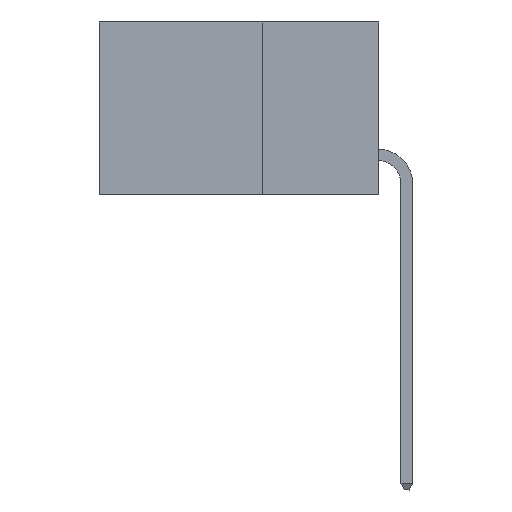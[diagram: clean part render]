
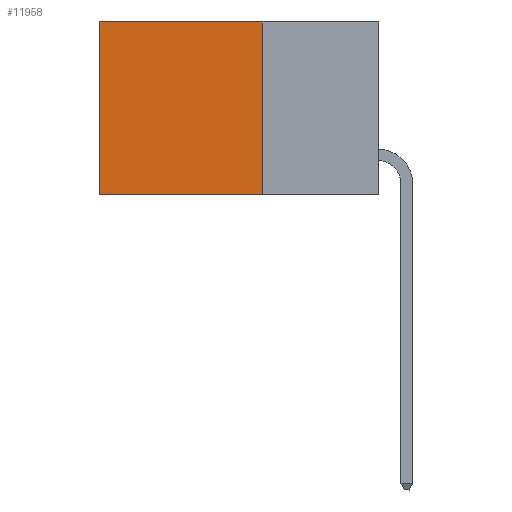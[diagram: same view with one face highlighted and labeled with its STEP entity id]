
A CAD part, left-side view. The second image highlights one B-rep face of the part: STEP entity #11958.
In plain terms, the highlighted planar face has unit normal (-1, 0, 0).
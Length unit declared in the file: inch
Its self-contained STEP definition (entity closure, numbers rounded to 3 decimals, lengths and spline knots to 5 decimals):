
#182 = DIRECTION ( 'NONE',  ( 0., 0., -1. ) ) ;
#1969 = CARTESIAN_POINT ( 'NONE',  ( 0.298, 0.25, -0.37 ) ) ;
#2810 = LINE ( 'NONE', #8745, #17818 ) ;
#3783 = CARTESIAN_POINT ( 'NONE',  ( 0.298, 0.25, 0. ) ) ;
#4049 = DIRECTION ( 'NONE',  ( 0., 1., 0. ) ) ;
#4136 = CARTESIAN_POINT ( 'NONE',  ( 0.298, 0.25, 0. ) ) ;
#6200 = DIRECTION ( 'NONE',  ( 0., 0., -1. ) ) ;
#7215 = VERTEX_POINT ( 'NONE', #12374 ) ;
#7547 = VECTOR ( 'NONE', #4049, 39.37008 ) ;
#8173 = VERTEX_POINT ( 'NONE', #13472 ) ;
#8325 = CARTESIAN_POINT ( 'NONE',  ( 0.298, 0.25, 0. ) ) ;
#8745 = CARTESIAN_POINT ( 'NONE',  ( 0.298, 0.6, 0. ) ) ;
#11142 = LINE ( 'NONE', #8325, #26065 ) ;
#11958 = ADVANCED_FACE ( 'NONE', ( #16698 ), #14303, .F. ) ;
#11993 = LINE ( 'NONE', #3783, #16780 ) ;
#12374 = CARTESIAN_POINT ( 'NONE',  ( 0.298, 0.6, 0. ) ) ;
#12513 = AXIS2_PLACEMENT_3D ( 'NONE', #4136, #18391, #6200 ) ;
#12549 = ORIENTED_EDGE ( 'NONE', *, *, #25322, .T. ) ;
#13472 = CARTESIAN_POINT ( 'NONE',  ( 0.298, 0.25, -0.37 ) ) ;
#14303 = PLANE ( 'NONE',  #12513 ) ;
#14525 = EDGE_CURVE ( 'NONE', #17636, #8173, #11142, .T. ) ;
#14815 = DIRECTION ( 'NONE',  ( 0., 0., -1. ) ) ;
#16698 = FACE_OUTER_BOUND ( 'NONE', #19529, .T. ) ;
#16713 = EDGE_CURVE ( 'NONE', #8173, #22495, #23759, .T. ) ;
#16772 = ORIENTED_EDGE ( 'NONE', *, *, #23159, .T. ) ;
#16780 = VECTOR ( 'NONE', #20055, 39.37008 ) ;
#17636 = VERTEX_POINT ( 'NONE', #23137 ) ;
#17818 = VECTOR ( 'NONE', #14815, 39.37008 ) ;
#18391 = DIRECTION ( 'NONE',  ( 1., 0., 0. ) ) ;
#18709 = ORIENTED_EDGE ( 'NONE', *, *, #14525, .F. ) ;
#19011 = CARTESIAN_POINT ( 'NONE',  ( 0.298, 0.6, -0.37 ) ) ;
#19529 = EDGE_LOOP ( 'NONE', ( #16772, #23924, #18709, #12549 ) ) ;
#20055 = DIRECTION ( 'NONE',  ( 0., 1., 0. ) ) ;
#22495 = VERTEX_POINT ( 'NONE', #19011 ) ;
#23137 = CARTESIAN_POINT ( 'NONE',  ( 0.298, 0.25, 0. ) ) ;
#23159 = EDGE_CURVE ( 'NONE', #7215, #22495, #2810, .T. ) ;
#23759 = LINE ( 'NONE', #1969, #7547 ) ;
#23924 = ORIENTED_EDGE ( 'NONE', *, *, #16713, .F. ) ;
#25322 = EDGE_CURVE ( 'NONE', #17636, #7215, #11993, .T. ) ;
#26065 = VECTOR ( 'NONE', #182, 39.37008 ) ;
